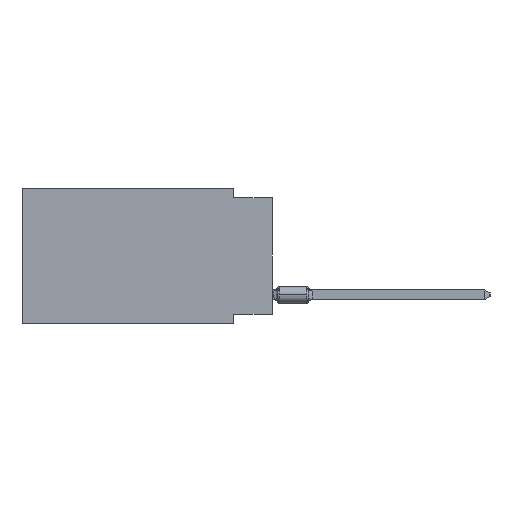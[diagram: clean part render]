
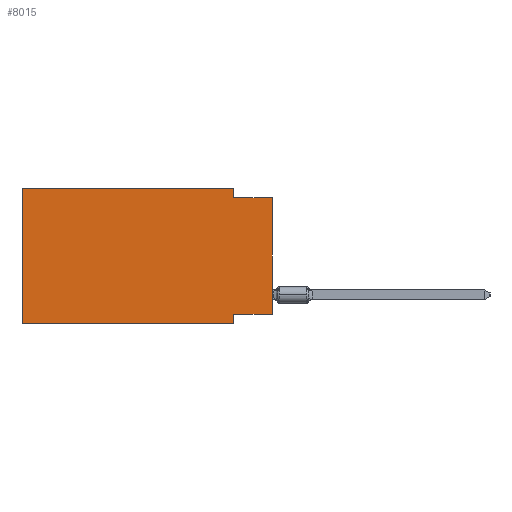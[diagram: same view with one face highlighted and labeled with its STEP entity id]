
A CAD part, left-side view. The second image highlights one B-rep face of the part: STEP entity #8015.
In plain terms, the highlighted planar face has unit normal (-1, 0, 0).
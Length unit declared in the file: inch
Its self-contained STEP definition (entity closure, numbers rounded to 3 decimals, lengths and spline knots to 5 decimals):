
#260 = AXIS2_PLACEMENT_3D ( 'NONE', #18541, #20152, #2335 ) ;
#547 = CARTESIAN_POINT ( 'NONE',  ( 0., 0.1, -0.325 ) ) ;
#652 = LINE ( 'NONE', #12032, #15840 ) ;
#715 = CARTESIAN_POINT ( 'NONE',  ( 0., 0.645, 0. ) ) ;
#952 = ORIENTED_EDGE ( 'NONE', *, *, #3065, .F. ) ;
#1165 = LINE ( 'NONE', #12739, #14355 ) ;
#2263 = ORIENTED_EDGE ( 'NONE', *, *, #14480, .F. ) ;
#2335 = DIRECTION ( 'NONE',  ( 0., 0., -1. ) ) ;
#3065 = EDGE_CURVE ( 'NONE', #14561, #8159, #8088, .T. ) ;
#3454 = VERTEX_POINT ( 'NONE', #11499 ) ;
#3747 = ORIENTED_EDGE ( 'NONE', *, *, #11268, .T. ) ;
#4476 = ORIENTED_EDGE ( 'NONE', *, *, #8143, .T. ) ;
#5452 = ORIENTED_EDGE ( 'NONE', *, *, #8633, .F. ) ;
#5551 = PLANE ( 'NONE',  #260 ) ;
#6091 = CARTESIAN_POINT ( 'NONE',  ( 0., 0.1, -0.025 ) ) ;
#6151 = CARTESIAN_POINT ( 'NONE',  ( 0., 0., -0.025 ) ) ;
#6883 = CARTESIAN_POINT ( 'NONE',  ( 0., 0.645, 0. ) ) ;
#7041 = VECTOR ( 'NONE', #16542, 39.37008 ) ;
#8015 = ADVANCED_FACE ( 'NONE', ( #17135 ), #5551, .F. ) ;
#8088 = LINE ( 'NONE', #11626, #7041 ) ;
#8143 = EDGE_CURVE ( 'NONE', #8563, #19573, #1165, .T. ) ;
#8159 = VERTEX_POINT ( 'NONE', #6091 ) ;
#8563 = VERTEX_POINT ( 'NONE', #9789 ) ;
#8633 = EDGE_CURVE ( 'NONE', #16684, #14561, #13316, .T. ) ;
#8724 = VERTEX_POINT ( 'NONE', #547 ) ;
#8814 = DIRECTION ( 'NONE',  ( 0., 0., -1. ) ) ;
#8949 = VECTOR ( 'NONE', #10723, 39.37008 ) ;
#9191 = CARTESIAN_POINT ( 'NONE',  ( 0., 0.645, 0. ) ) ;
#9224 = LINE ( 'NONE', #15546, #8949 ) ;
#9525 = ORIENTED_EDGE ( 'NONE', *, *, #9616, .F. ) ;
#9616 = EDGE_CURVE ( 'NONE', #8159, #3454, #16430, .T. ) ;
#9665 = LINE ( 'NONE', #12987, #16088 ) ;
#9789 = CARTESIAN_POINT ( 'NONE',  ( 0., 0.645, -0.35 ) ) ;
#10584 = DIRECTION ( 'NONE',  ( 0., 0., 1. ) ) ;
#10723 = DIRECTION ( 'NONE',  ( 0., 1., 0. ) ) ;
#10867 = ORIENTED_EDGE ( 'NONE', *, *, #11983, .F. ) ;
#11268 = EDGE_CURVE ( 'NONE', #16792, #3454, #9665, .T. ) ;
#11386 = DIRECTION ( 'NONE',  ( 0., 0., 1. ) ) ;
#11499 = CARTESIAN_POINT ( 'NONE',  ( 0., 0., -0.025 ) ) ;
#11626 = CARTESIAN_POINT ( 'NONE',  ( 0., 0.1, 0. ) ) ;
#11819 = DIRECTION ( 'NONE',  ( 0., -1., 0. ) ) ;
#11983 = EDGE_CURVE ( 'NONE', #8563, #16684, #15301, .T. ) ;
#12032 = CARTESIAN_POINT ( 'NONE',  ( 0., 0.1, -0.35 ) ) ;
#12255 = CARTESIAN_POINT ( 'NONE',  ( 0., 0., -0.325 ) ) ;
#12739 = CARTESIAN_POINT ( 'NONE',  ( 0., 0.645, -0.35 ) ) ;
#12752 = EDGE_CURVE ( 'NONE', #16792, #8724, #9224, .T. ) ;
#12987 = CARTESIAN_POINT ( 'NONE',  ( 0., 0., 0. ) ) ;
#13316 = LINE ( 'NONE', #6883, #16075 ) ;
#13572 = ORIENTED_EDGE ( 'NONE', *, *, #12752, .F. ) ;
#13643 = CARTESIAN_POINT ( 'NONE',  ( 0., 0.1, 0. ) ) ;
#14190 = CARTESIAN_POINT ( 'NONE',  ( 0., 0.1, -0.35 ) ) ;
#14355 = VECTOR ( 'NONE', #17787, 39.37008 ) ;
#14480 = EDGE_CURVE ( 'NONE', #8724, #19573, #652, .T. ) ;
#14561 = VERTEX_POINT ( 'NONE', #13643 ) ;
#15301 = LINE ( 'NONE', #715, #16774 ) ;
#15546 = CARTESIAN_POINT ( 'NONE',  ( 0., 0., -0.325 ) ) ;
#15840 = VECTOR ( 'NONE', #8814, 39.37008 ) ;
#16075 = VECTOR ( 'NONE', #11819, 39.37008 ) ;
#16088 = VECTOR ( 'NONE', #11386, 39.37008 ) ;
#16430 = LINE ( 'NONE', #6151, #19175 ) ;
#16542 = DIRECTION ( 'NONE',  ( 0., 0., -1. ) ) ;
#16684 = VERTEX_POINT ( 'NONE', #9191 ) ;
#16774 = VECTOR ( 'NONE', #10584, 39.37008 ) ;
#16792 = VERTEX_POINT ( 'NONE', #12255 ) ;
#17135 = FACE_OUTER_BOUND ( 'NONE', #19666, .T. ) ;
#17787 = DIRECTION ( 'NONE',  ( 0., -1., 0. ) ) ;
#18541 = CARTESIAN_POINT ( 'NONE',  ( 0., 0.645, 0. ) ) ;
#19175 = VECTOR ( 'NONE', #21159, 39.37008 ) ;
#19573 = VERTEX_POINT ( 'NONE', #14190 ) ;
#19666 = EDGE_LOOP ( 'NONE', ( #3747, #9525, #952, #5452, #10867, #4476, #2263, #13572 ) ) ;
#20152 = DIRECTION ( 'NONE',  ( 1., 0., 0. ) ) ;
#21159 = DIRECTION ( 'NONE',  ( 0., -1., 0. ) ) ;
